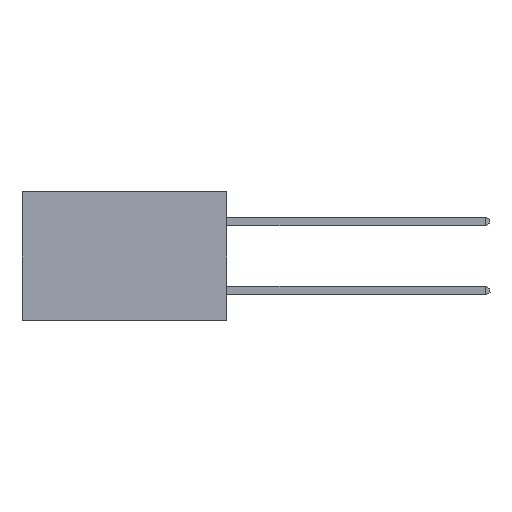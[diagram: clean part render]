
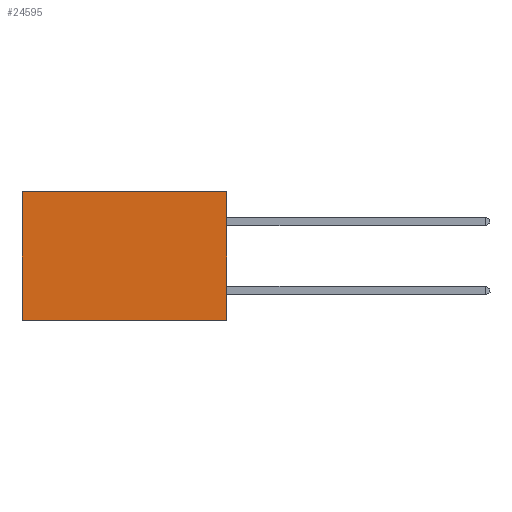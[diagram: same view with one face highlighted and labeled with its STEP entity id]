
A CAD part, left-side view. The second image highlights one B-rep face of the part: STEP entity #24595.
In plain terms, the highlighted planar face has unit normal (-1, 0, 0).
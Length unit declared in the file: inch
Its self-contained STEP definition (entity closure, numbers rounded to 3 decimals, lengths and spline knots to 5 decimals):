
#2856 = DIRECTION ( 'NONE',  ( 0., 1., 0. ) ) ;
#2923 = ORIENTED_EDGE ( 'NONE', *, *, #7930, .F. ) ;
#3830 = LINE ( 'NONE', #5078, #14890 ) ;
#3950 = FACE_OUTER_BOUND ( 'NONE', #7439, .T. ) ;
#4140 = PLANE ( 'NONE',  #21339 ) ;
#4347 = VECTOR ( 'NONE', #18195, 39.37008 ) ;
#5078 = CARTESIAN_POINT ( 'NONE',  ( 0.277, 0., 0. ) ) ;
#5397 = VECTOR ( 'NONE', #15370, 39.37008 ) ;
#6363 = ORIENTED_EDGE ( 'NONE', *, *, #24124, .T. ) ;
#7076 = CARTESIAN_POINT ( 'NONE',  ( 0.277, 0.59, -0.37 ) ) ;
#7439 = EDGE_LOOP ( 'NONE', ( #6363, #22086, #2923, #27618 ) ) ;
#7802 = CARTESIAN_POINT ( 'NONE',  ( 0.277, 0., 0. ) ) ;
#7930 = EDGE_CURVE ( 'NONE', #19281, #20173, #22665, .T. ) ;
#10839 = CARTESIAN_POINT ( 'NONE',  ( 0.277, 0., -0.37 ) ) ;
#11285 = LINE ( 'NONE', #7076, #22320 ) ;
#13036 = DIRECTION ( 'NONE',  ( 0., 0., -1. ) ) ;
#13506 = CARTESIAN_POINT ( 'NONE',  ( 0.277, 0.59, 0. ) ) ;
#14890 = VECTOR ( 'NONE', #2856, 39.37008 ) ;
#15370 = DIRECTION ( 'NONE',  ( 0., 1., 0. ) ) ;
#16866 = EDGE_CURVE ( 'NONE', #20173, #18187, #28163, .T. ) ;
#17612 = CARTESIAN_POINT ( 'NONE',  ( 0.277, 0.59, -0.37 ) ) ;
#18187 = VERTEX_POINT ( 'NONE', #17612 ) ;
#18195 = DIRECTION ( 'NONE',  ( 0., 0., -1. ) ) ;
#19281 = VERTEX_POINT ( 'NONE', #7802 ) ;
#19458 = CARTESIAN_POINT ( 'NONE',  ( 0.277, 0., -0.37 ) ) ;
#20173 = VERTEX_POINT ( 'NONE', #19458 ) ;
#20877 = EDGE_CURVE ( 'NONE', #19281, #22782, #3830, .T. ) ;
#21339 = AXIS2_PLACEMENT_3D ( 'NONE', #10839, #26259, #13036 ) ;
#22086 = ORIENTED_EDGE ( 'NONE', *, *, #16866, .F. ) ;
#22320 = VECTOR ( 'NONE', #26947, 39.37008 ) ;
#22470 = CARTESIAN_POINT ( 'NONE',  ( 0.277, 0., -0.37 ) ) ;
#22665 = LINE ( 'NONE', #24799, #4347 ) ;
#22782 = VERTEX_POINT ( 'NONE', #13506 ) ;
#24124 = EDGE_CURVE ( 'NONE', #22782, #18187, #11285, .T. ) ;
#24595 = ADVANCED_FACE ( 'NONE', ( #3950 ), #4140, .F. ) ;
#24799 = CARTESIAN_POINT ( 'NONE',  ( 0.277, 0., -0.37 ) ) ;
#26259 = DIRECTION ( 'NONE',  ( 1., 0., 0. ) ) ;
#26947 = DIRECTION ( 'NONE',  ( 0., 0., -1. ) ) ;
#27618 = ORIENTED_EDGE ( 'NONE', *, *, #20877, .T. ) ;
#28163 = LINE ( 'NONE', #22470, #5397 ) ;
